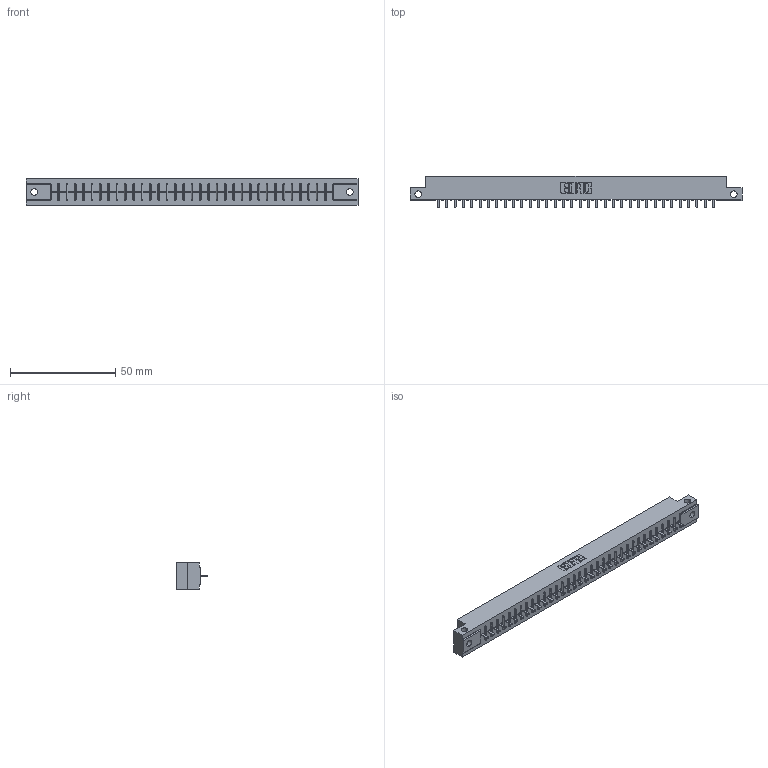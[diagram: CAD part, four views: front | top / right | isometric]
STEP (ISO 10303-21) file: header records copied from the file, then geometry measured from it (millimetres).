
FILE_DESCRIPTION (( 'STEP AP203' ), '1' );
FILE_NAME ('306-034-421-112.STEP', '2020-09-22T03:33:34', ( '' ), ( '' ), 'SwSTEP 2.0', 'SolidWorks 2020', '' );
FILE_SCHEMA (( 'CONFIG_CONTROL_DESIGN' ));
Length unit declared in the file: inch
Products named in the file (3): 306 Part_.128 Dia; 306-034-421-112; 306-290-001_121
Assembly tree (35 placements, depth 2):
  306-034-421-112
    306 Part_.128 Dia
    306-290-001_121  x34
Bounding box: 157.73 x 14.88 x 12.7 mm (x, y, z)
Volume: 17123.3 mm3; surface area: 17279.6 mm2
Topology: 35 solids, 35 shells, 2508 faces, 7050 edges, 4512 vertices
Faces by surface type: plane 1666, cylinder 706, sphere 136
Entity records: 33105 total; most frequent: CARTESIAN_POINT 5605, ORIENTED_EDGE 5512, DIRECTION 5466, EDGE_CURVE 2756, VECTOR 2136, LINE 2136, VERTEX_POINT 1740, AXIS2_PLACEMENT_3D 1665
